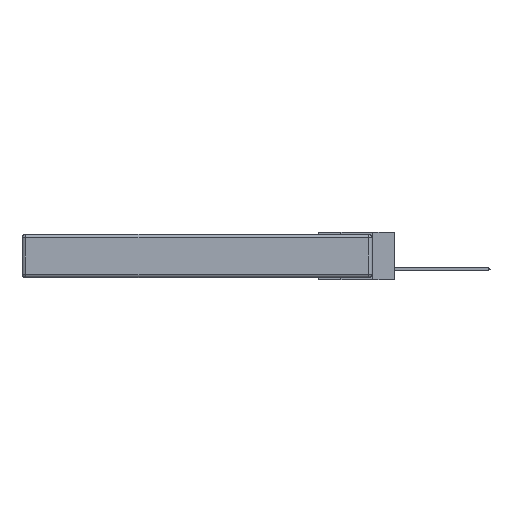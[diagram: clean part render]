
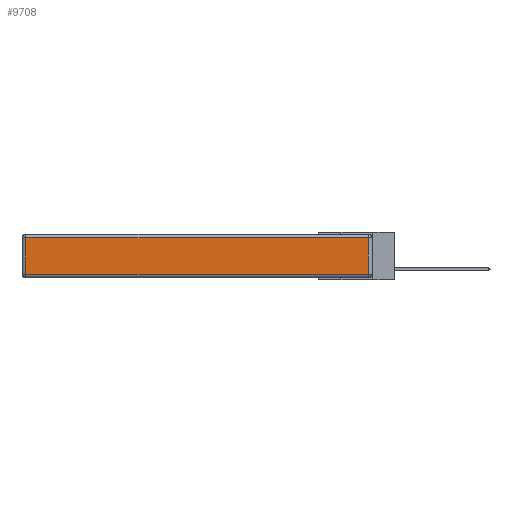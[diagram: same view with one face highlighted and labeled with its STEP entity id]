
A CAD part, left-side view. The second image highlights one B-rep face of the part: STEP entity #9708.
In plain terms, the highlighted planar face has unit normal (-1, 0, 0).
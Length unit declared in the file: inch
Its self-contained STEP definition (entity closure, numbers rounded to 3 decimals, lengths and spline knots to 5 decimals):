
#422 = DIRECTION ( 'NONE',  ( 0., 0., 1. ) ) ;
#726 = LINE ( 'NONE', #25745, #5336 ) ;
#909 = VECTOR ( 'NONE', #15558, 39.37008 ) ;
#1065 = CARTESIAN_POINT ( 'NONE',  ( 0., 0., -0.313 ) ) ;
#2203 = VERTEX_POINT ( 'NONE', #13804 ) ;
#2559 = EDGE_LOOP ( 'NONE', ( #21366, #23312, #13083, #24919 ) ) ;
#2928 = VECTOR ( 'NONE', #422, 39.37008 ) ;
#4481 = EDGE_CURVE ( 'NONE', #2203, #17617, #17615, .T. ) ;
#4878 = DIRECTION ( 'NONE',  ( 0., 1., 0. ) ) ;
#5336 = VECTOR ( 'NONE', #23705, 39.37008 ) ;
#6486 = CARTESIAN_POINT ( 'NONE',  ( 0., 0.03, -0.343 ) ) ;
#7027 = EDGE_CURVE ( 'NONE', #17617, #7126, #726, .T. ) ;
#7126 = VERTEX_POINT ( 'NONE', #17787 ) ;
#8245 = EDGE_CURVE ( 'NONE', #9920, #2203, #14111, .T. ) ;
#9642 = EDGE_CURVE ( 'NONE', #7126, #9920, #21883, .T. ) ;
#9708 = ADVANCED_FACE ( 'NONE', ( #21243 ), #10457, .T. ) ;
#9920 = VERTEX_POINT ( 'NONE', #12345 ) ;
#10457 = PLANE ( 'NONE',  #11784 ) ;
#11784 = AXIS2_PLACEMENT_3D ( 'NONE', #21088, #25011, #16785 ) ;
#12345 = CARTESIAN_POINT ( 'NONE',  ( 0., 0.03, -0.313 ) ) ;
#13083 = ORIENTED_EDGE ( 'NONE', *, *, #4481, .T. ) ;
#13787 = CARTESIAN_POINT ( 'NONE',  ( 0., 2.72, -0.03 ) ) ;
#13804 = CARTESIAN_POINT ( 'NONE',  ( 0., 0.03, -0.03 ) ) ;
#14111 = LINE ( 'NONE', #6486, #2928 ) ;
#15558 = DIRECTION ( 'NONE',  ( 0., -1., 0. ) ) ;
#16785 = DIRECTION ( 'NONE',  ( 0., 0., 1. ) ) ;
#17615 = LINE ( 'NONE', #23734, #22489 ) ;
#17617 = VERTEX_POINT ( 'NONE', #13787 ) ;
#17787 = CARTESIAN_POINT ( 'NONE',  ( 0., 2.72, -0.313 ) ) ;
#21088 = CARTESIAN_POINT ( 'NONE',  ( 0., 0., -0.343 ) ) ;
#21243 = FACE_OUTER_BOUND ( 'NONE', #2559, .T. ) ;
#21366 = ORIENTED_EDGE ( 'NONE', *, *, #9642, .T. ) ;
#21883 = LINE ( 'NONE', #1065, #909 ) ;
#22489 = VECTOR ( 'NONE', #4878, 39.37008 ) ;
#23312 = ORIENTED_EDGE ( 'NONE', *, *, #8245, .T. ) ;
#23705 = DIRECTION ( 'NONE',  ( 0., 0., -1. ) ) ;
#23734 = CARTESIAN_POINT ( 'NONE',  ( 0., 2.75, -0.03 ) ) ;
#24919 = ORIENTED_EDGE ( 'NONE', *, *, #7027, .T. ) ;
#25011 = DIRECTION ( 'NONE',  ( -1., 0., 0. ) ) ;
#25745 = CARTESIAN_POINT ( 'NONE',  ( 0., 2.72, -0.343 ) ) ;
